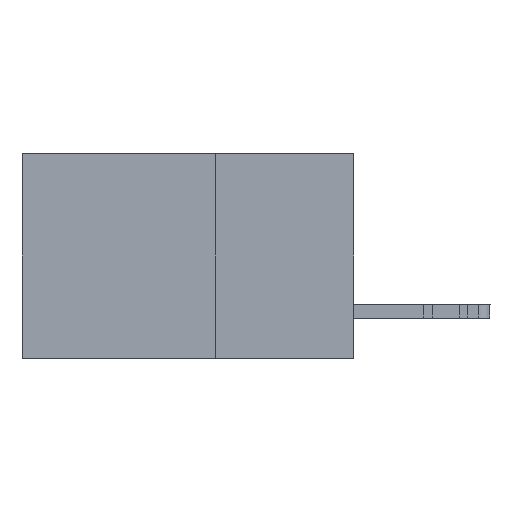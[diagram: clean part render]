
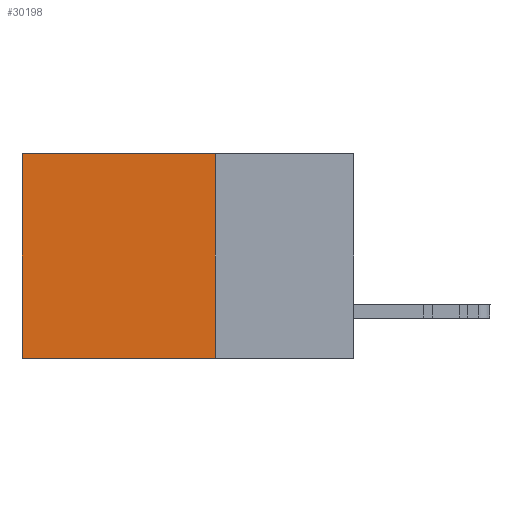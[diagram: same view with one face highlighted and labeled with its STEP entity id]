
A CAD part, left-side view. The second image highlights one B-rep face of the part: STEP entity #30198.
In plain terms, the highlighted planar face has unit normal (-1, 0, 0).
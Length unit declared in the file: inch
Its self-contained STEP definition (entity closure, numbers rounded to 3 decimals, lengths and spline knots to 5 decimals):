
#284 = VERTEX_POINT ( 'NONE', #3906 ) ;
#1315 = LINE ( 'NONE', #23134, #7170 ) ;
#1443 = CARTESIAN_POINT ( 'NONE',  ( 0.2875, 0.25, 0. ) ) ;
#1929 = ORIENTED_EDGE ( 'NONE', *, *, #10454, .F. ) ;
#3695 = LINE ( 'NONE', #36508, #16041 ) ;
#3906 = CARTESIAN_POINT ( 'NONE',  ( 0.2875, 0.6, -0.37 ) ) ;
#4547 = VERTEX_POINT ( 'NONE', #10802 ) ;
#7170 = VECTOR ( 'NONE', #46176, 39.37008 ) ;
#10403 = ORIENTED_EDGE ( 'NONE', *, *, #24018, .T. ) ;
#10454 = EDGE_CURVE ( 'NONE', #29613, #284, #3695, .T. ) ;
#10802 = CARTESIAN_POINT ( 'NONE',  ( 0.2875, 0.6, 0. ) ) ;
#12483 = ORIENTED_EDGE ( 'NONE', *, *, #31241, .T. ) ;
#13014 = FACE_OUTER_BOUND ( 'NONE', #13604, .T. ) ;
#13604 = EDGE_LOOP ( 'NONE', ( #12483, #1929, #36198, #10403 ) ) ;
#13880 = DIRECTION ( 'NONE',  ( 0., 1., 0. ) ) ;
#14070 = LINE ( 'NONE', #39338, #20640 ) ;
#15669 = VECTOR ( 'NONE', #24590, 39.37008 ) ;
#16041 = VECTOR ( 'NONE', #13880, 39.37008 ) ;
#16817 = PLANE ( 'NONE',  #18381 ) ;
#18381 = AXIS2_PLACEMENT_3D ( 'NONE', #27545, #42082, #23510 ) ;
#19994 = EDGE_CURVE ( 'NONE', #42073, #29613, #25055, .T. ) ;
#20640 = VECTOR ( 'NONE', #20994, 39.37008 ) ;
#20994 = DIRECTION ( 'NONE',  ( 0., 0., -1. ) ) ;
#23134 = CARTESIAN_POINT ( 'NONE',  ( 0.2875, 0.25, 0. ) ) ;
#23510 = DIRECTION ( 'NONE',  ( 0., 0., -1. ) ) ;
#24018 = EDGE_CURVE ( 'NONE', #42073, #4547, #1315, .T. ) ;
#24590 = DIRECTION ( 'NONE',  ( 0., 0., -1. ) ) ;
#25055 = LINE ( 'NONE', #35567, #15669 ) ;
#27545 = CARTESIAN_POINT ( 'NONE',  ( 0.2875, 0.25, 0. ) ) ;
#29613 = VERTEX_POINT ( 'NONE', #46350 ) ;
#30198 = ADVANCED_FACE ( 'NONE', ( #13014 ), #16817, .F. ) ;
#31241 = EDGE_CURVE ( 'NONE', #4547, #284, #14070, .T. ) ;
#35567 = CARTESIAN_POINT ( 'NONE',  ( 0.2875, 0.25, 0. ) ) ;
#36198 = ORIENTED_EDGE ( 'NONE', *, *, #19994, .F. ) ;
#36508 = CARTESIAN_POINT ( 'NONE',  ( 0.2875, 0.25, -0.37 ) ) ;
#39338 = CARTESIAN_POINT ( 'NONE',  ( 0.2875, 0.6, 0. ) ) ;
#42073 = VERTEX_POINT ( 'NONE', #1443 ) ;
#42082 = DIRECTION ( 'NONE',  ( 1., 0., 0. ) ) ;
#46176 = DIRECTION ( 'NONE',  ( 0., 1., 0. ) ) ;
#46350 = CARTESIAN_POINT ( 'NONE',  ( 0.2875, 0.25, -0.37 ) ) ;
